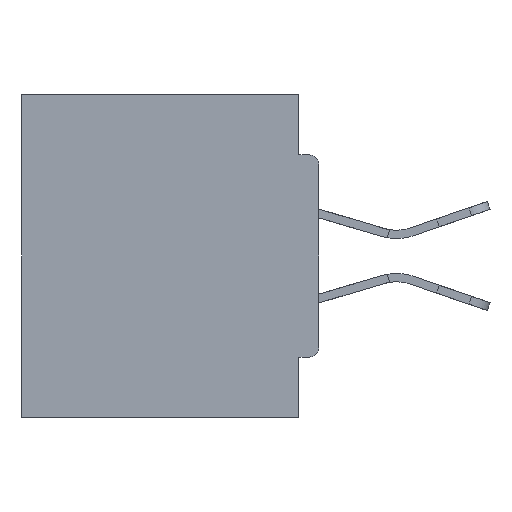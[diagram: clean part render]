
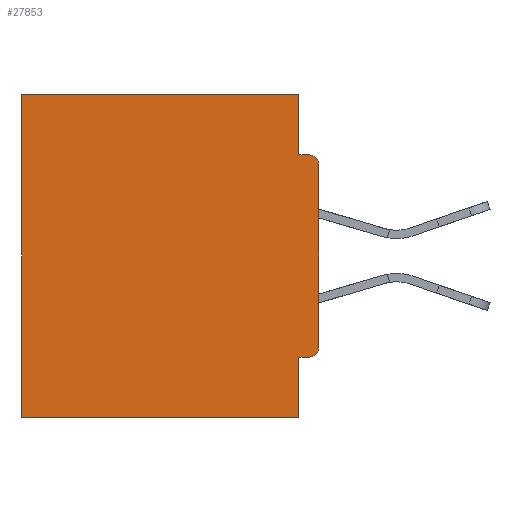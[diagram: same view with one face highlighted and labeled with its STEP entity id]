
A CAD part, left-side view. The second image highlights one B-rep face of the part: STEP entity #27853.
In plain terms, the highlighted planar face has unit normal (-1, 0, 0).
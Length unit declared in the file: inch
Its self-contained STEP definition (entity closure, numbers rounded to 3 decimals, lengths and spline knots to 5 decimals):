
#641 = VERTEX_POINT ( 'NONE', #16467 ) ;
#2189 = LINE ( 'NONE', #20253, #19332 ) ;
#2233 = CARTESIAN_POINT ( 'NONE',  ( 0.298, 0.46, 0. ) ) ;
#2748 = DIRECTION ( 'NONE',  ( 0., 0., -1. ) ) ;
#2808 = DIRECTION ( 'NONE',  ( 0., -1., 0. ) ) ;
#3176 = CARTESIAN_POINT ( 'NONE',  ( 0.298, 0., 0. ) ) ;
#3260 = DIRECTION ( 'NONE',  ( 0., 0., -1. ) ) ;
#3632 = LINE ( 'NONE', #28131, #29615 ) ;
#3815 = EDGE_CURVE ( 'NONE', #30755, #641, #19975, .T. ) ;
#4887 = CIRCLE ( 'NONE', #24843, 0.015 ) ;
#4993 = EDGE_CURVE ( 'NONE', #37057, #13200, #40319, .T. ) ;
#5959 = LINE ( 'NONE', #11362, #20896 ) ;
#6116 = AXIS2_PLACEMENT_3D ( 'NONE', #3176, #42462, #13687 ) ;
#6880 = PLANE ( 'NONE',  #6116 ) ;
#6890 = CARTESIAN_POINT ( 'NONE',  ( 0.298, 0.015, -0.1085 ) ) ;
#7881 = ORIENTED_EDGE ( 'NONE', *, *, #4993, .F. ) ;
#8338 = ORIENTED_EDGE ( 'NONE', *, *, #3815, .F. ) ;
#8451 = ORIENTED_EDGE ( 'NONE', *, *, #36653, .T. ) ;
#8560 = CARTESIAN_POINT ( 'NONE',  ( 0.298, 0.015, -0.4065 ) ) ;
#9098 = EDGE_CURVE ( 'NONE', #37057, #34808, #24005, .T. ) ;
#10237 = AXIS2_PLACEMENT_3D ( 'NONE', #18055, #35577, #42812 ) ;
#11174 = VERTEX_POINT ( 'NONE', #34800 ) ;
#11362 = CARTESIAN_POINT ( 'NONE',  ( 0.298, 0.031, -0.5 ) ) ;
#11521 = DIRECTION ( 'NONE',  ( 0., 0., -1. ) ) ;
#12949 = EDGE_CURVE ( 'NONE', #40483, #19210, #4887, .T. ) ;
#12962 = LINE ( 'NONE', #45670, #19562 ) ;
#12998 = CARTESIAN_POINT ( 'NONE',  ( 0.298, 0.015, -0.0935 ) ) ;
#13200 = VERTEX_POINT ( 'NONE', #28246 ) ;
#13469 = EDGE_CURVE ( 'NONE', #11174, #30755, #5959, .T. ) ;
#13687 = DIRECTION ( 'NONE',  ( 0., 0., -1. ) ) ;
#15064 = CARTESIAN_POINT ( 'NONE',  ( 0.298, 0., -0.3915 ) ) ;
#15099 = CARTESIAN_POINT ( 'NONE',  ( 0.298, 0.031, 0. ) ) ;
#15133 = EDGE_CURVE ( 'NONE', #40483, #21773, #44615, .T. ) ;
#15161 = VECTOR ( 'NONE', #33322, 39.37008 ) ;
#15652 = DIRECTION ( 'NONE',  ( 0., 1., 0. ) ) ;
#16467 = CARTESIAN_POINT ( 'NONE',  ( 0.298, 0.46, -0.5 ) ) ;
#16664 = ORIENTED_EDGE ( 'NONE', *, *, #12949, .T. ) ;
#17541 = CIRCLE ( 'NONE', #10237, 0.015 ) ;
#18055 = CARTESIAN_POINT ( 'NONE',  ( 0.298, 0.015, -0.3915 ) ) ;
#18077 = FACE_OUTER_BOUND ( 'NONE', #30957, .T. ) ;
#19210 = VERTEX_POINT ( 'NONE', #12998 ) ;
#19332 = VECTOR ( 'NONE', #2808, 39.37008 ) ;
#19562 = VECTOR ( 'NONE', #3260, 39.37008 ) ;
#19975 = LINE ( 'NONE', #39970, #41049 ) ;
#20253 = CARTESIAN_POINT ( 'NONE',  ( 0.298, 0., -0.0935 ) ) ;
#20896 = VECTOR ( 'NONE', #43414, 39.37008 ) ;
#21773 = VERTEX_POINT ( 'NONE', #15064 ) ;
#22045 = ORIENTED_EDGE ( 'NONE', *, *, #29096, .F. ) ;
#22164 = ORIENTED_EDGE ( 'NONE', *, *, #15133, .F. ) ;
#23311 = VERTEX_POINT ( 'NONE', #8560 ) ;
#23680 = VECTOR ( 'NONE', #28442, 39.37008 ) ;
#23858 = DIRECTION ( 'NONE',  ( -1., 0., 0. ) ) ;
#24005 = LINE ( 'NONE', #29583, #15161 ) ;
#24843 = AXIS2_PLACEMENT_3D ( 'NONE', #6890, #23858, #2748 ) ;
#27496 = EDGE_CURVE ( 'NONE', #23311, #21773, #17541, .T. ) ;
#27853 = ADVANCED_FACE ( 'NONE', ( #18077 ), #6880, .F. ) ;
#28131 = CARTESIAN_POINT ( 'NONE',  ( 0.298, 0., -0.4065 ) ) ;
#28246 = CARTESIAN_POINT ( 'NONE',  ( 0.298, 0.031, -0.0935 ) ) ;
#28442 = DIRECTION ( 'NONE',  ( 0., 0., -1. ) ) ;
#29047 = CARTESIAN_POINT ( 'NONE',  ( 0.298, 0.031, -0.5 ) ) ;
#29096 = EDGE_CURVE ( 'NONE', #23311, #11174, #3632, .T. ) ;
#29583 = CARTESIAN_POINT ( 'NONE',  ( 0.298, 0., 0. ) ) ;
#29615 = VECTOR ( 'NONE', #31765, 39.37008 ) ;
#29987 = ORIENTED_EDGE ( 'NONE', *, *, #13469, .F. ) ;
#30755 = VERTEX_POINT ( 'NONE', #29047 ) ;
#30957 = EDGE_LOOP ( 'NONE', ( #16664, #37182, #7881, #31212, #8451, #8338, #29987, #22045, #41002, #22164 ) ) ;
#31212 = ORIENTED_EDGE ( 'NONE', *, *, #9098, .T. ) ;
#31765 = DIRECTION ( 'NONE',  ( 0., 1., 0. ) ) ;
#33322 = DIRECTION ( 'NONE',  ( 0., 1., 0. ) ) ;
#33461 = EDGE_CURVE ( 'NONE', #13200, #19210, #2189, .T. ) ;
#33527 = VECTOR ( 'NONE', #11521, 39.37008 ) ;
#34800 = CARTESIAN_POINT ( 'NONE',  ( 0.298, 0.031, -0.4065 ) ) ;
#34808 = VERTEX_POINT ( 'NONE', #2233 ) ;
#35296 = CARTESIAN_POINT ( 'NONE',  ( 0.298, 0., -0.1085 ) ) ;
#35577 = DIRECTION ( 'NONE',  ( -1., 0., 0. ) ) ;
#36653 = EDGE_CURVE ( 'NONE', #34808, #641, #12962, .T. ) ;
#37057 = VERTEX_POINT ( 'NONE', #15099 ) ;
#37182 = ORIENTED_EDGE ( 'NONE', *, *, #33461, .F. ) ;
#38877 = CARTESIAN_POINT ( 'NONE',  ( 0.298, 0.031, -0.5 ) ) ;
#39552 = CARTESIAN_POINT ( 'NONE',  ( 0.298, 0., 0. ) ) ;
#39970 = CARTESIAN_POINT ( 'NONE',  ( 0.298, 0., -0.5 ) ) ;
#40319 = LINE ( 'NONE', #38877, #23680 ) ;
#40483 = VERTEX_POINT ( 'NONE', #35296 ) ;
#41002 = ORIENTED_EDGE ( 'NONE', *, *, #27496, .T. ) ;
#41049 = VECTOR ( 'NONE', #15652, 39.37008 ) ;
#42462 = DIRECTION ( 'NONE',  ( 1., 0., 0. ) ) ;
#42812 = DIRECTION ( 'NONE',  ( 0., 0., -1. ) ) ;
#43414 = DIRECTION ( 'NONE',  ( 0., 0., -1. ) ) ;
#44615 = LINE ( 'NONE', #39552, #33527 ) ;
#45670 = CARTESIAN_POINT ( 'NONE',  ( 0.298, 0.46, 0. ) ) ;
